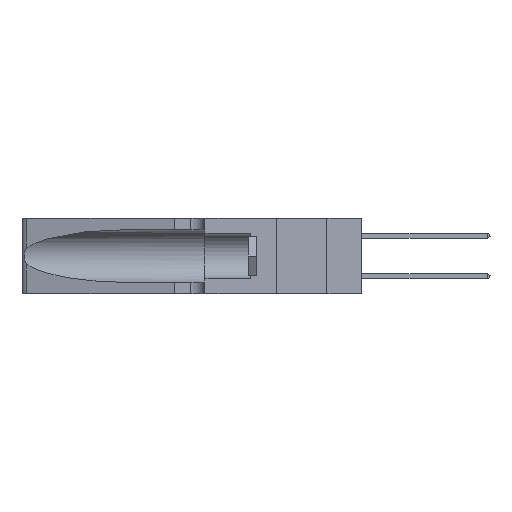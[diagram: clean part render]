
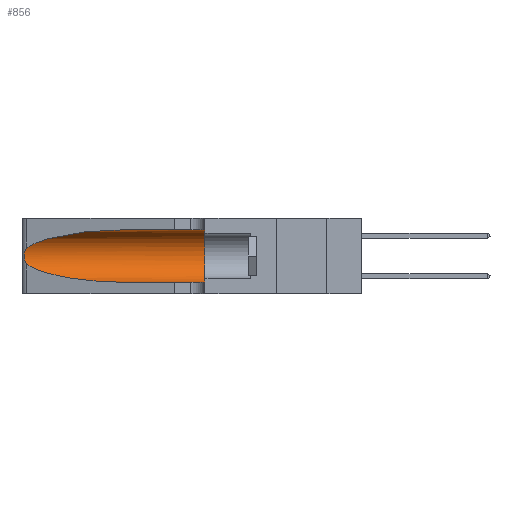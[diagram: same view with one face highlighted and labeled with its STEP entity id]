
A CAD part, left-side view. The second image highlights one B-rep face of the part: STEP entity #856.
In plain terms, the highlighted cylindrical face has radius 3.308 mm (diameter 6.617 mm), a partial arc.
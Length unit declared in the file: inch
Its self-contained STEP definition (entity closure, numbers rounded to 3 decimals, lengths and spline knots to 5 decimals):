
#856 = ADVANCED_FACE ( 'NONE', ( #3368 ), #9696, .F. ) ;
#1261 = CARTESIAN_POINT ( 'NONE',  ( 0.25487, 1.22718, 0.14631 ) ) ;
#1661 = CARTESIAN_POINT ( 'NONE',  ( 0.25487, 1.22718, 0.22369 ) ) ;
#2590 = CARTESIAN_POINT ( 'NONE',  ( 0.25487, 1.22718, 0.14631 ) ) ;
#2771 = CARTESIAN_POINT ( 'NONE',  ( 0.1305, 0.35, 0.05475 ) ) ;
#2786 = CARTESIAN_POINT ( 'NONE',  ( 0.25487, 1.22718, 0.22369 ) ) ;
#3029 = DIRECTION ( 'NONE',  ( 0., -1., 0. ) ) ;
#3368 = FACE_OUTER_BOUND ( 'NONE', #8282, .T. ) ;
#3763 = CARTESIAN_POINT ( 'NONE',  ( 0.26017, 1.23833, 0.17102 ) ) ;
#4395 = CARTESIAN_POINT ( 'NONE',  ( 0.1305, 0.72297, 0.31525 ) ) ;
#4957 = CARTESIAN_POINT ( 'NONE',  ( 0.1305, 1.61858, 0.31525 ) ) ;
#5002 = VERTEX_POINT ( 'NONE', #7999 ) ;
#5279 = ORIENTED_EDGE ( 'NONE', *, *, #12048, .T. ) ;
#5648 = VERTEX_POINT ( 'NONE', #2771 ) ;
#5741 = AXIS2_PLACEMENT_3D ( 'NONE', #16305, #6812, #18203 ) ;
#5784 = CARTESIAN_POINT ( 'NONE',  ( 0.25639, 1.23184, 0.21858 ) ) ;
#5865 = CARTESIAN_POINT ( 'NONE',  ( 0.25555, 1.22994, 0.2215 ) ) ;
#6003 = DIRECTION ( 'NONE',  ( 0., 0., 1. ) ) ;
#6091 = CARTESIAN_POINT ( 'NONE',  ( 0.25487, 1.22718, 0.22369 ) ) ;
#6812 = DIRECTION ( 'NONE',  ( 0., -1., 0. ) ) ;
#7877 = VERTEX_POINT ( 'NONE', #2590 ) ;
#7965 = CARTESIAN_POINT ( 'NONE',  ( 0.26018, 1.23835, 0.19895 ) ) ;
#7999 = CARTESIAN_POINT ( 'NONE',  ( 0.1305, 0.35, 0.31525 ) ) ;
#8112 = CARTESIAN_POINT ( 'NONE',  ( 0.1305, 0.35, 0.185 ) ) ;
#8223 = CIRCLE ( 'NONE', #22790, 0.13025 ) ;
#8282 = EDGE_LOOP ( 'NONE', ( #15212, #5279, #8309, #16560, #8934, #21947 ) ) ;
#8309 = ORIENTED_EDGE ( 'NONE', *, *, #20016, .T. ) ;
#8615 = VECTOR ( 'NONE', #3029, 39.37008 ) ;
#8934 = ORIENTED_EDGE ( 'NONE', *, *, #10737, .F. ) ;
#8970 = VERTEX_POINT ( 'NONE', #10624 ) ;
#8976 = EDGE_CURVE ( 'NONE', #10160, #5648, #16397, .T. ) ;
#9696 = CYLINDRICAL_SURFACE ( 'NONE', #5741, 0.13025 ) ;
#10127 = EDGE_CURVE ( 'NONE', #8970, #23574, #13288, .T. ) ;
#10160 = VERTEX_POINT ( 'NONE', #14498 ) ;
#10624 = CARTESIAN_POINT ( 'NONE',  ( 0.1305, 0.72297, 0.31525 ) ) ;
#10737 = EDGE_CURVE ( 'NONE', #5002, #5648, #8223, .T. ) ;
#10959 = CARTESIAN_POINT ( 'NONE',  ( 0.18966, 0.96281, 0.05475 ) ) ;
#11771 = CARTESIAN_POINT ( 'NONE',  ( 0.25787, 1.23484, 0.2124 ) ) ;
#12020 = CARTESIAN_POINT ( 'NONE',  ( 0.25639, 1.23186, 0.15144 ) ) ;
#12048 = EDGE_CURVE ( 'NONE', #23574, #7877, #21153, .T. ) ;
#12098 = CARTESIAN_POINT ( 'NONE',  ( 0.25856, 1.23593, 0.16098 ) ) ;
#12442 = CARTESIAN_POINT ( 'NONE',  ( 0.25555, 1.22993, 0.14849 ) ) ;
#13288 =( BOUNDED_CURVE ( )  B_SPLINE_CURVE ( 3, ( #4395, #15745, #19805, #6091 ),
 .UNSPECIFIED., .F., .F. ) 
 B_SPLINE_CURVE_WITH_KNOTS ( ( 4, 4 ),
 ( 1.5708, 2.84003 ),
 .UNSPECIFIED. ) 
 CURVE ( )  GEOMETRIC_REPRESENTATION_ITEM ( )  RATIONAL_B_SPLINE_CURVE ( ( 1., 0.87, 0.87, 1. ) ) 
 REPRESENTATION_ITEM ( '' )  );
#13749 = CARTESIAN_POINT ( 'NONE',  ( 0.26075, 1.23896, 0.19203 ) ) ;
#13901 = DIRECTION ( 'NONE',  ( 0., 1., 0. ) ) ;
#14213 = DIRECTION ( 'NONE',  ( 0., -1., 0. ) ) ;
#14498 = CARTESIAN_POINT ( 'NONE',  ( 0.1305, 0.72297, 0.05475 ) ) ;
#14647 = LINE ( 'NONE', #4957, #8615 ) ;
#14896 = VECTOR ( 'NONE', #14213, 39.37008 ) ;
#15212 = ORIENTED_EDGE ( 'NONE', *, *, #10127, .T. ) ;
#15275 = CARTESIAN_POINT ( 'NONE',  ( 0.26075, 1.23896, 0.178 ) ) ;
#15745 = CARTESIAN_POINT ( 'NONE',  ( 0.18966, 0.96281, 0.31525 ) ) ;
#16122 = CARTESIAN_POINT ( 'NONE',  ( 0.25487, 1.22718, 0.14631 ) ) ;
#16305 = CARTESIAN_POINT ( 'NONE',  ( 0.1305, 1.61858, 0.185 ) ) ;
#16397 = LINE ( 'NONE', #20115, #14896 ) ;
#16560 = ORIENTED_EDGE ( 'NONE', *, *, #8976, .T. ) ;
#18203 = DIRECTION ( 'NONE',  ( 0., 0., -1. ) ) ;
#19490 = CARTESIAN_POINT ( 'NONE',  ( 0.25854, 1.2359, 0.20912 ) ) ;
#19805 = CARTESIAN_POINT ( 'NONE',  ( 0.2373, 1.15595, 0.28018 ) ) ;
#20016 = EDGE_CURVE ( 'NONE', #7877, #10160, #22699, .T. ) ;
#20115 = CARTESIAN_POINT ( 'NONE',  ( 0.1305, 1.61858, 0.05475 ) ) ;
#20681 = CARTESIAN_POINT ( 'NONE',  ( 0.2373, 1.15595, 0.08982 ) ) ;
#21153 = B_SPLINE_CURVE_WITH_KNOTS ( 'NONE', 3,
 ( #1661, #5865, #5784, #11771, #19490, #7965, #13749, #15275, #3763, #12098, #21757, #12020, #12442, #16122 ),
 .UNSPECIFIED., .F., .F.,
 ( 4, 2, 2, 2, 2, 2, 4 ),
 ( 0., 0.00027, 0.00053, 0.00107, 0.0016, 0.00187, 0.00214 ),
 .UNSPECIFIED. ) ;
#21757 = CARTESIAN_POINT ( 'NONE',  ( 0.25789, 1.23486, 0.15765 ) ) ;
#21947 = ORIENTED_EDGE ( 'NONE', *, *, #23672, .F. ) ;
#22699 =( BOUNDED_CURVE ( )  B_SPLINE_CURVE ( 3, ( #1261, #20681, #10959, #24371 ),
 .UNSPECIFIED., .F., .F. ) 
 B_SPLINE_CURVE_WITH_KNOTS ( ( 4, 4 ),
 ( 3.44316, 4.71239 ),
 .UNSPECIFIED. ) 
 CURVE ( )  GEOMETRIC_REPRESENTATION_ITEM ( )  RATIONAL_B_SPLINE_CURVE ( ( 1., 0.87, 0.87, 1. ) ) 
 REPRESENTATION_ITEM ( '' )  );
#22790 = AXIS2_PLACEMENT_3D ( 'NONE', #8112, #13901, #6003 ) ;
#23574 = VERTEX_POINT ( 'NONE', #2786 ) ;
#23672 = EDGE_CURVE ( 'NONE', #8970, #5002, #14647, .T. ) ;
#24371 = CARTESIAN_POINT ( 'NONE',  ( 0.1305, 0.72297, 0.05475 ) ) ;
